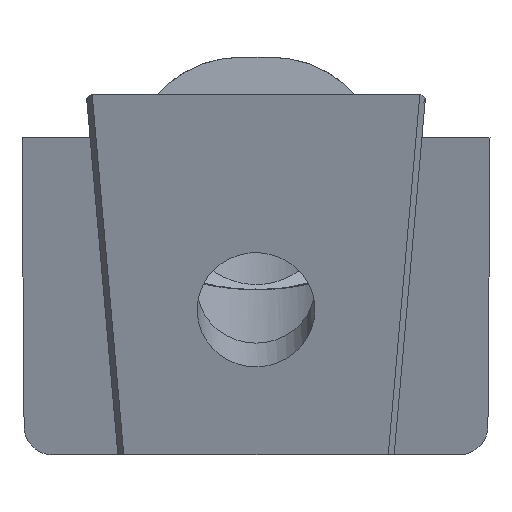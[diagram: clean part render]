
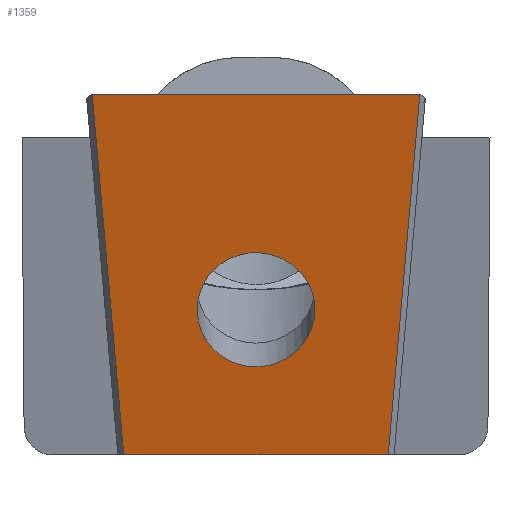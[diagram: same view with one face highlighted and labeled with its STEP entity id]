
A CAD part, front view. The second image highlights one B-rep face of the part: STEP entity #1359.
In plain terms, the highlighted planar face has unit normal (0, -0.966, -0.259).
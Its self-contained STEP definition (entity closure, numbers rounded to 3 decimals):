
#46=ELLIPSE('',#1498,2.079,2.075);
#125=LINE('',#2401,#227);
#146=LINE('',#2767,#248);
#147=LINE('',#2769,#249);
#148=LINE('',#2770,#250);
#227=VECTOR('',#1701,10.);
#248=VECTOR('',#1826,10.);
#249=VECTOR('',#1827,10.);
#250=VECTOR('',#1828,10.);
#289=FACE_BOUND('',#422,.T.);
#341=FACE_OUTER_BOUND('',#421,.T.);
#421=EDGE_LOOP('',(#1130,#1131,#1132,#1133));
#422=EDGE_LOOP('',(#1134));
#600=VERTEX_POINT('',#2398);
#601=VERTEX_POINT('',#2400);
#638=VERTEX_POINT('',#2757);
#639=VERTEX_POINT('',#2766);
#640=VERTEX_POINT('',#2768);
#754=EDGE_CURVE('',#601,#600,#125,.T.);
#814=EDGE_CURVE('',#638,#638,#46,.T.);
#818=EDGE_CURVE('',#639,#600,#146,.T.);
#819=EDGE_CURVE('',#639,#640,#147,.T.);
#820=EDGE_CURVE('',#601,#640,#148,.T.);
#1130=ORIENTED_EDGE('',*,*,#818,.F.);
#1131=ORIENTED_EDGE('',*,*,#819,.T.);
#1132=ORIENTED_EDGE('',*,*,#820,.F.);
#1133=ORIENTED_EDGE('',*,*,#754,.T.);
#1134=ORIENTED_EDGE('',*,*,#814,.T.);
#1295=PLANE('',#1503);
#1359=ADVANCED_FACE('',(#341,#289),#1295,.T.);
#1498=AXIS2_PLACEMENT_3D('',#2758,#1812,#1813);
#1503=AXIS2_PLACEMENT_3D('',#2765,#1824,#1825);
#1701=DIRECTION('',(-1.,0.,0.));
#1812=DIRECTION('center_axis',(0.,0.966,0.259));
#1813=DIRECTION('ref_axis',(0.,0.259,-0.966));
#1824=DIRECTION('center_axis',(0.,-0.966,-0.259));
#1825=DIRECTION('ref_axis',(-1.,0.,0.));
#1826=DIRECTION('',(-0.084,-0.258,0.962));
#1827=DIRECTION('',(1.,0.,0.));
#1828=DIRECTION('',(-0.084,0.258,-0.962));
#2398=CARTESIAN_POINT('',(-12.246,134.01,12.697));
#2400=CARTESIAN_POINT('',(-0.714,134.01,12.697));
#2401=CARTESIAN_POINT('',(0.998,134.01,12.697));
#2757=CARTESIAN_POINT('',(-4.405,136.043,5.108));
#2758=CARTESIAN_POINT('Origin',(-6.48,136.043,5.108));
#2765=CARTESIAN_POINT('Origin',(-1.524,137.412,0.));
#2766=CARTESIAN_POINT('',(-11.135,137.412,0.));
#2767=CARTESIAN_POINT('',(-11.102,137.514,-0.379));
#2768=CARTESIAN_POINT('',(-1.825,137.412,0.));
#2769=CARTESIAN_POINT('',(0.248,137.412,0.));
#2770=CARTESIAN_POINT('',(-1.853,137.497,-0.319));
